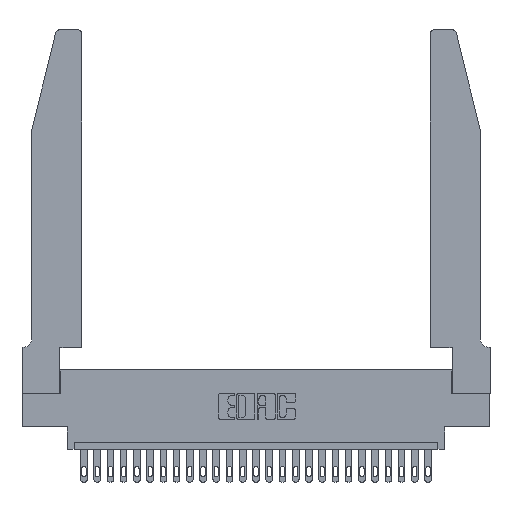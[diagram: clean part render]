
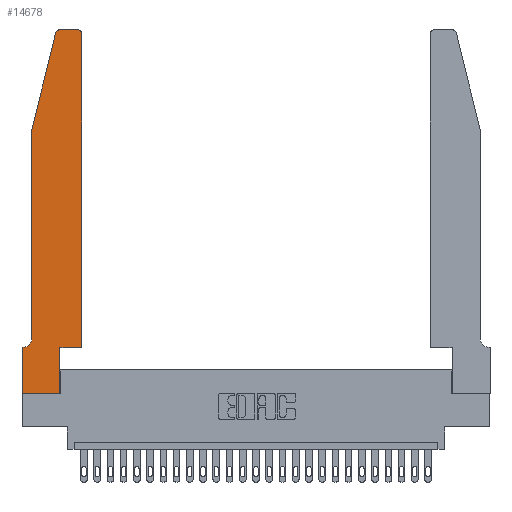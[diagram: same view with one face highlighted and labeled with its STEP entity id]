
A CAD part, top view. The second image highlights one B-rep face of the part: STEP entity #14678.
In plain terms, the highlighted planar face has unit normal (0, 0, 1).
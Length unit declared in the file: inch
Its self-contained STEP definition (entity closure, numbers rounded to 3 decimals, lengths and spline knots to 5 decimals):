
#272 = LINE ( 'NONE', #22009, #20552 ) ;
#658 = VECTOR ( 'NONE', #22186, 39.37008 ) ;
#730 = DIRECTION ( 'NONE',  ( 0., 0., 1. ) ) ;
#1425 = VERTEX_POINT ( 'NONE', #22342 ) ;
#2355 = LINE ( 'NONE', #7346, #23981 ) ;
#2565 = CARTESIAN_POINT ( 'NONE',  ( 0.4505, 0.35, 0.37 ) ) ;
#2765 = DIRECTION ( 'NONE',  ( 1., 0., 0. ) ) ;
#2847 = DIRECTION ( 'NONE',  ( 1., 0., 0. ) ) ;
#3310 = PLANE ( 'NONE',  #8215 ) ;
#3335 = DIRECTION ( 'NONE',  ( -1., 0., 0. ) ) ;
#3430 = EDGE_CURVE ( 'NONE', #14054, #18778, #22305, .T. ) ;
#3436 = EDGE_CURVE ( 'NONE', #1425, #4294, #23280, .T. ) ;
#3490 = DIRECTION ( 'NONE',  ( 0., 0., 1. ) ) ;
#3578 = AXIS2_PLACEMENT_3D ( 'NONE', #23810, #7343, #13665 ) ;
#3978 = CARTESIAN_POINT ( 'NONE',  ( 0., 0., 0.37 ) ) ;
#4294 = VERTEX_POINT ( 'NONE', #3978 ) ;
#4369 = LINE ( 'NONE', #13790, #26648 ) ;
#5617 = ORIENTED_EDGE ( 'NONE', *, *, #3430, .T. ) ;
#6251 = ORIENTED_EDGE ( 'NONE', *, *, #19338, .T. ) ;
#6819 = CARTESIAN_POINT ( 'NONE',  ( 0.284, 2.72, 0.37 ) ) ;
#6842 = VERTEX_POINT ( 'NONE', #16540 ) ;
#7343 = DIRECTION ( 'NONE',  ( 0., 0., -1. ) ) ;
#7346 = CARTESIAN_POINT ( 'NONE',  ( 0.2605, 2.75, 0.37 ) ) ;
#7388 = CARTESIAN_POINT ( 'NONE',  ( 0.0755, 0.35, 0.37 ) ) ;
#7459 = DIRECTION ( 'NONE',  ( 0., -1., 0. ) ) ;
#7513 = ORIENTED_EDGE ( 'NONE', *, *, #9877, .T. ) ;
#7549 = LINE ( 'NONE', #7388, #19252 ) ;
#7575 = VECTOR ( 'NONE', #12604, 39.37008 ) ;
#7962 = VERTEX_POINT ( 'NONE', #11904 ) ;
#8208 = VECTOR ( 'NONE', #24532, 39.37008 ) ;
#8215 = AXIS2_PLACEMENT_3D ( 'NONE', #22021, #3490, #24646 ) ;
#9752 = VECTOR ( 'NONE', #7459, 39.37008 ) ;
#9877 = EDGE_CURVE ( 'NONE', #7962, #6842, #4369, .T. ) ;
#10041 = VERTEX_POINT ( 'NONE', #15213 ) ;
#10431 = VERTEX_POINT ( 'NONE', #2565 ) ;
#10923 = VERTEX_POINT ( 'NONE', #11535 ) ;
#11242 = EDGE_CURVE ( 'NONE', #20164, #10923, #23297, .T. ) ;
#11526 = CARTESIAN_POINT ( 'NONE',  ( 0.0755, 2., 0.37 ) ) ;
#11535 = CARTESIAN_POINT ( 'NONE',  ( 0.0055, 0.35, 0.37 ) ) ;
#11904 = CARTESIAN_POINT ( 'NONE',  ( 0.2865, 0., 0.37 ) ) ;
#12376 = ORIENTED_EDGE ( 'NONE', *, *, #15693, .T. ) ;
#12604 = DIRECTION ( 'NONE',  ( 0., 1., 0. ) ) ;
#12918 = ORIENTED_EDGE ( 'NONE', *, *, #16797, .T. ) ;
#13286 = CARTESIAN_POINT ( 'NONE',  ( 0.4205, 2.72, 0.37 ) ) ;
#13665 = DIRECTION ( 'NONE',  ( -1., 0., 0. ) ) ;
#13790 = CARTESIAN_POINT ( 'NONE',  ( 0.2865, 0.35, 0.37 ) ) ;
#14054 = VERTEX_POINT ( 'NONE', #20820 ) ;
#14079 = CARTESIAN_POINT ( 'NONE',  ( 0.0755, 0.42, 0.37 ) ) ;
#14653 = EDGE_CURVE ( 'NONE', #17212, #22064, #17079, .T. ) ;
#14678 = ADVANCED_FACE ( 'NONE', ( #16738 ), #3310, .T. ) ;
#14986 = EDGE_CURVE ( 'NONE', #18778, #10041, #2355, .T. ) ;
#15095 = ORIENTED_EDGE ( 'NONE', *, *, #14653, .T. ) ;
#15213 = CARTESIAN_POINT ( 'NONE',  ( 0.284, 2.75, 0.37 ) ) ;
#15614 = ORIENTED_EDGE ( 'NONE', *, *, #11242, .T. ) ;
#15693 = EDGE_CURVE ( 'NONE', #4294, #7962, #18302, .T. ) ;
#16540 = CARTESIAN_POINT ( 'NONE',  ( 0.2865, 0.35, 0.37 ) ) ;
#16738 = FACE_OUTER_BOUND ( 'NONE', #23191, .T. ) ;
#16797 = EDGE_CURVE ( 'NONE', #22064, #20164, #27155, .T. ) ;
#17079 = LINE ( 'NONE', #17830, #26955 ) ;
#17113 = DIRECTION ( 'NONE',  ( -1., 0., 0. ) ) ;
#17212 = VERTEX_POINT ( 'NONE', #25281 ) ;
#17830 = CARTESIAN_POINT ( 'NONE',  ( 0.0755, 2., 0.37 ) ) ;
#18211 = DIRECTION ( 'NONE',  ( 0., 1., 0. ) ) ;
#18302 = LINE ( 'NONE', #26195, #8208 ) ;
#18778 = VERTEX_POINT ( 'NONE', #25516 ) ;
#19078 = AXIS2_PLACEMENT_3D ( 'NONE', #6819, #19661, #19382 ) ;
#19252 = VECTOR ( 'NONE', #3335, 39.37008 ) ;
#19338 = EDGE_CURVE ( 'NONE', #10041, #17212, #23173, .T. ) ;
#19382 = DIRECTION ( 'NONE',  ( 1., 0., 0. ) ) ;
#19661 = DIRECTION ( 'NONE',  ( 0., 0., 1. ) ) ;
#20164 = VERTEX_POINT ( 'NONE', #14079 ) ;
#20552 = VECTOR ( 'NONE', #2765, 39.37008 ) ;
#20643 = ORIENTED_EDGE ( 'NONE', *, *, #24173, .T. ) ;
#20820 = CARTESIAN_POINT ( 'NONE',  ( 0.4505, 2.72, 0.37 ) ) ;
#20875 = ORIENTED_EDGE ( 'NONE', *, *, #14986, .T. ) ;
#21109 = AXIS2_PLACEMENT_3D ( 'NONE', #13286, #730, #2847 ) ;
#21779 = ORIENTED_EDGE ( 'NONE', *, *, #23775, .T. ) ;
#21935 = DIRECTION ( 'NONE',  ( -0.239, -0.971, 0. ) ) ;
#22009 = CARTESIAN_POINT ( 'NONE',  ( 0.4505, 0.35, 0.37 ) ) ;
#22021 = CARTESIAN_POINT ( 'NONE',  ( 0., 0.35, 0.37 ) ) ;
#22064 = VERTEX_POINT ( 'NONE', #11526 ) ;
#22186 = DIRECTION ( 'NONE',  ( 0., -1., 0. ) ) ;
#22305 = CIRCLE ( 'NONE', #21109, 0.03 ) ;
#22342 = CARTESIAN_POINT ( 'NONE',  ( 0., 0.35, 0.37 ) ) ;
#23173 = CIRCLE ( 'NONE', #19078, 0.03 ) ;
#23191 = EDGE_LOOP ( 'NONE', ( #20875, #6251, #15095, #12918, #15614, #20643, #27001, #12376, #7513, #25645, #21779, #5617 ) ) ;
#23280 = LINE ( 'NONE', #25836, #658 ) ;
#23297 = CIRCLE ( 'NONE', #3578, 0.07 ) ;
#23775 = EDGE_CURVE ( 'NONE', #10431, #14054, #24256, .T. ) ;
#23810 = CARTESIAN_POINT ( 'NONE',  ( 0.0055, 0.42, 0.37 ) ) ;
#23981 = VECTOR ( 'NONE', #17113, 39.37008 ) ;
#24173 = EDGE_CURVE ( 'NONE', #10923, #1425, #7549, .T. ) ;
#24256 = LINE ( 'NONE', #25149, #7575 ) ;
#24532 = DIRECTION ( 'NONE',  ( 1., 0., 0. ) ) ;
#24646 = DIRECTION ( 'NONE',  ( 1., 0., 0. ) ) ;
#24685 = EDGE_CURVE ( 'NONE', #6842, #10431, #272, .T. ) ;
#25149 = CARTESIAN_POINT ( 'NONE',  ( 0.4505, 0.35, 0.37 ) ) ;
#25281 = CARTESIAN_POINT ( 'NONE',  ( 0.25487, 2.72718, 0.37 ) ) ;
#25516 = CARTESIAN_POINT ( 'NONE',  ( 0.4205, 2.75, 0.37 ) ) ;
#25645 = ORIENTED_EDGE ( 'NONE', *, *, #24685, .T. ) ;
#25836 = CARTESIAN_POINT ( 'NONE',  ( 0., 0., 0.37 ) ) ;
#26131 = CARTESIAN_POINT ( 'NONE',  ( 0.0755, 2., 0.37 ) ) ;
#26195 = CARTESIAN_POINT ( 'NONE',  ( 0., 0., 0.37 ) ) ;
#26648 = VECTOR ( 'NONE', #18211, 39.37008 ) ;
#26955 = VECTOR ( 'NONE', #21935, 39.37008 ) ;
#27001 = ORIENTED_EDGE ( 'NONE', *, *, #3436, .T. ) ;
#27155 = LINE ( 'NONE', #26131, #9752 ) ;
